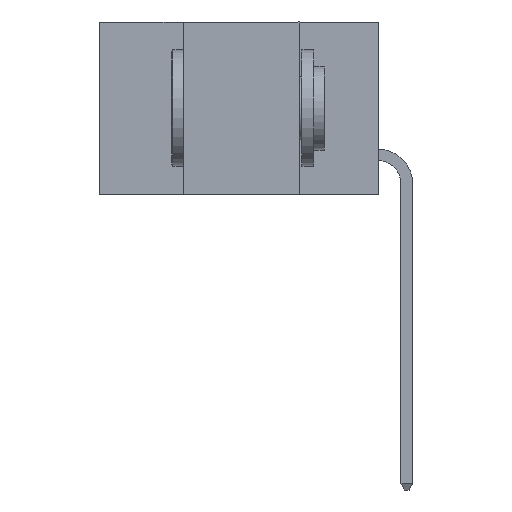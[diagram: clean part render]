
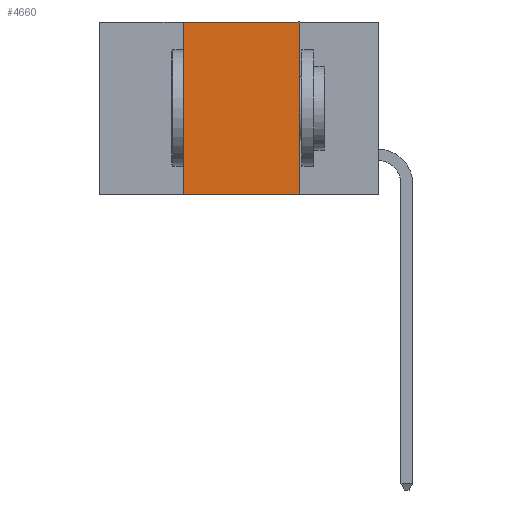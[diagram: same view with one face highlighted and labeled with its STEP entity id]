
A CAD part, left-side view. The second image highlights one B-rep face of the part: STEP entity #4660.
In plain terms, the highlighted planar face has unit normal (-1, 0, 0).
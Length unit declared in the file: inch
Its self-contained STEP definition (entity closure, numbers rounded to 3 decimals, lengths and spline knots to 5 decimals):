
#127 = FACE_OUTER_BOUND ( 'NONE', #9138, .T. ) ;
#624 = VERTEX_POINT ( 'NONE', #8699 ) ;
#901 = LINE ( 'NONE', #2997, #5660 ) ;
#994 = DIRECTION ( 'NONE',  ( 1., 0., 0. ) ) ;
#1510 = VERTEX_POINT ( 'NONE', #7726 ) ;
#1759 = DIRECTION ( 'NONE',  ( 0., 0., 1. ) ) ;
#2163 = EDGE_CURVE ( 'NONE', #624, #1510, #9060, .T. ) ;
#2189 = CARTESIAN_POINT ( 'NONE',  ( 0., 0.42, -0.37 ) ) ;
#2732 = DIRECTION ( 'NONE',  ( 0., 0., -1. ) ) ;
#2838 = EDGE_CURVE ( 'NONE', #624, #7160, #10495, .T. ) ;
#2880 = DIRECTION ( 'NONE',  ( 0., 0., -1. ) ) ;
#2997 = CARTESIAN_POINT ( 'NONE',  ( 0., 0.17, -0.37 ) ) ;
#3033 = CARTESIAN_POINT ( 'NONE',  ( 0., 0.6, 0. ) ) ;
#3088 = ORIENTED_EDGE ( 'NONE', *, *, #2838, .F. ) ;
#3214 = PLANE ( 'NONE',  #7829 ) ;
#4093 = VECTOR ( 'NONE', #10377, 39.37008 ) ;
#4169 = EDGE_CURVE ( 'NONE', #7160, #8548, #4412, .T. ) ;
#4412 = LINE ( 'NONE', #10399, #4093 ) ;
#4660 = ADVANCED_FACE ( 'NONE', ( #127 ), #3214, .F. ) ;
#4829 = EDGE_CURVE ( 'NONE', #8548, #1510, #901, .T. ) ;
#5660 = VECTOR ( 'NONE', #2880, 39.37008 ) ;
#7160 = VERTEX_POINT ( 'NONE', #9009 ) ;
#7726 = CARTESIAN_POINT ( 'NONE',  ( 0., 0.17, -0.37 ) ) ;
#7783 = VECTOR ( 'NONE', #1759, 39.37008 ) ;
#7812 = ORIENTED_EDGE ( 'NONE', *, *, #4829, .F. ) ;
#7829 = AXIS2_PLACEMENT_3D ( 'NONE', #3033, #994, #2732 ) ;
#7983 = CARTESIAN_POINT ( 'NONE',  ( 0., 0.17, 0. ) ) ;
#8128 = ORIENTED_EDGE ( 'NONE', *, *, #4169, .F. ) ;
#8548 = VERTEX_POINT ( 'NONE', #7983 ) ;
#8699 = CARTESIAN_POINT ( 'NONE',  ( 0., 0.42, -0.37 ) ) ;
#9009 = CARTESIAN_POINT ( 'NONE',  ( 0., 0.42, 0. ) ) ;
#9060 = LINE ( 'NONE', #9643, #9394 ) ;
#9138 = EDGE_LOOP ( 'NONE', ( #7812, #8128, #3088, #11800 ) ) ;
#9394 = VECTOR ( 'NONE', #9741, 39.37008 ) ;
#9643 = CARTESIAN_POINT ( 'NONE',  ( 0., 0.6, -0.37 ) ) ;
#9741 = DIRECTION ( 'NONE',  ( 0., -1., 0. ) ) ;
#10377 = DIRECTION ( 'NONE',  ( 0., -1., 0. ) ) ;
#10399 = CARTESIAN_POINT ( 'NONE',  ( 0., 0.6, 0. ) ) ;
#10495 = LINE ( 'NONE', #2189, #7783 ) ;
#11800 = ORIENTED_EDGE ( 'NONE', *, *, #2163, .T. ) ;
